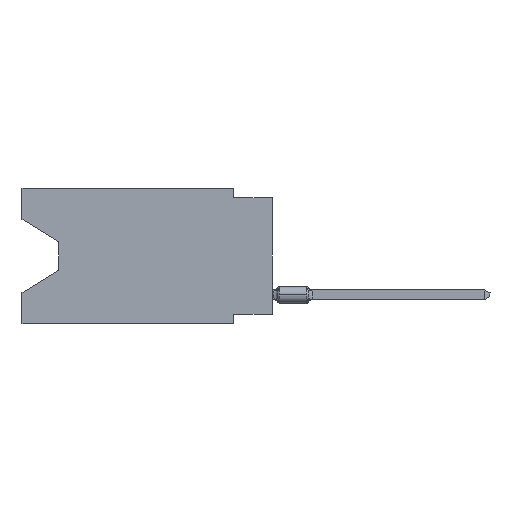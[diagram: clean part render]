
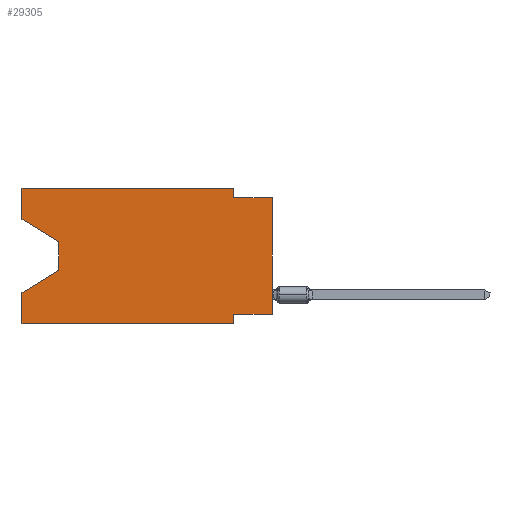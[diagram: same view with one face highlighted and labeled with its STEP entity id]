
A CAD part, left-side view. The second image highlights one B-rep face of the part: STEP entity #29305.
In plain terms, the highlighted planar face has unit normal (-1, 0, 0).
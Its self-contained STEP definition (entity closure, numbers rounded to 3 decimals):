
#318 = DIRECTION ( 'NONE',  ( 0., 0., -1. ) ) ;
#501 = VERTEX_POINT ( 'NONE', #9343 ) ;
#638 = CARTESIAN_POINT ( 'NONE',  ( 0., 0., -8.255 ) ) ;
#1353 = LINE ( 'NONE', #30160, #41318 ) ;
#1791 = VERTEX_POINT ( 'NONE', #24906 ) ;
#1804 = VERTEX_POINT ( 'NONE', #42028 ) ;
#1901 = VECTOR ( 'NONE', #5568, 1000. ) ;
#2150 = ORIENTED_EDGE ( 'NONE', *, *, #16579, .F. ) ;
#2250 = EDGE_CURVE ( 'NONE', #501, #45289, #46612, .T. ) ;
#2260 = CARTESIAN_POINT ( 'NONE',  ( 0., 0., 0. ) ) ;
#2474 = LINE ( 'NONE', #16874, #13094 ) ;
#3110 = DIRECTION ( 'NONE',  ( 1., 0., 0. ) ) ;
#3567 = LINE ( 'NONE', #17994, #26788 ) ;
#4320 = EDGE_CURVE ( 'NONE', #13395, #40575, #29215, .T. ) ;
#4702 = VECTOR ( 'NONE', #33225, 1000. ) ;
#4953 = CARTESIAN_POINT ( 'NONE',  ( 0., 2.54, -8.89 ) ) ;
#5279 = ORIENTED_EDGE ( 'NONE', *, *, #11830, .F. ) ;
#5568 = DIRECTION ( 'NONE',  ( 0., 0., 1. ) ) ;
#6064 = CARTESIAN_POINT ( 'NONE',  ( 0., 0., -8.255 ) ) ;
#6344 = CARTESIAN_POINT ( 'NONE',  ( 0., 16.383, -8.89 ) ) ;
#7563 = VECTOR ( 'NONE', #28225, 1000. ) ;
#7940 = DIRECTION ( 'NONE',  ( 0., 1., 0. ) ) ;
#8797 = VECTOR ( 'NONE', #27141, 1000. ) ;
#9343 = CARTESIAN_POINT ( 'NONE',  ( 0., 16.383, -2.038 ) ) ;
#9358 = DIRECTION ( 'NONE',  ( 0., 0.855, -0.519 ) ) ;
#10024 = LINE ( 'NONE', #21334, #24580 ) ;
#10184 = VECTOR ( 'NONE', #20744, 1000. ) ;
#10785 = DIRECTION ( 'NONE',  ( 0., 0., -1. ) ) ;
#11239 = ORIENTED_EDGE ( 'NONE', *, *, #15817, .F. ) ;
#11830 = EDGE_CURVE ( 'NONE', #44606, #1804, #18575, .T. ) ;
#12514 = CARTESIAN_POINT ( 'NONE',  ( 0., 16.383, 0. ) ) ;
#13094 = VECTOR ( 'NONE', #14985, 1000. ) ;
#13395 = VERTEX_POINT ( 'NONE', #42194 ) ;
#13863 = CARTESIAN_POINT ( 'NONE',  ( 0., 2.54, -8.89 ) ) ;
#13986 = FACE_OUTER_BOUND ( 'NONE', #30178, .T. ) ;
#14334 = AXIS2_PLACEMENT_3D ( 'NONE', #35450, #3110, #39457 ) ;
#14600 = EDGE_CURVE ( 'NONE', #44606, #38113, #16658, .T. ) ;
#14623 = EDGE_CURVE ( 'NONE', #40575, #28723, #3567, .T. ) ;
#14646 = ORIENTED_EDGE ( 'NONE', *, *, #37536, .F. ) ;
#14985 = DIRECTION ( 'NONE',  ( 0., -1., 0. ) ) ;
#15817 = EDGE_CURVE ( 'NONE', #28723, #38113, #2474, .T. ) ;
#16579 = EDGE_CURVE ( 'NONE', #1804, #25787, #42405, .T. ) ;
#16658 = LINE ( 'NONE', #2260, #1901 ) ;
#16874 = CARTESIAN_POINT ( 'NONE',  ( 0., 0., -0.635 ) ) ;
#17994 = CARTESIAN_POINT ( 'NONE',  ( 0., 2.54, 0. ) ) ;
#18475 = ORIENTED_EDGE ( 'NONE', *, *, #20558, .T. ) ;
#18575 = LINE ( 'NONE', #638, #31846 ) ;
#19889 = LINE ( 'NONE', #44659, #41288 ) ;
#20558 = EDGE_CURVE ( 'NONE', #45289, #23572, #10024, .T. ) ;
#20721 = ORIENTED_EDGE ( 'NONE', *, *, #4320, .F. ) ;
#20744 = DIRECTION ( 'NONE',  ( 0., -1., 0. ) ) ;
#21334 = CARTESIAN_POINT ( 'NONE',  ( 0., 13.97, -3.505 ) ) ;
#21909 = CARTESIAN_POINT ( 'NONE',  ( 0., 16.383, 0. ) ) ;
#23572 = VERTEX_POINT ( 'NONE', #41243 ) ;
#24580 = VECTOR ( 'NONE', #318, 1000. ) ;
#24906 = CARTESIAN_POINT ( 'NONE',  ( 0., 16.383, -8.89 ) ) ;
#24958 = EDGE_CURVE ( 'NONE', #501, #13395, #26904, .T. ) ;
#25787 = VERTEX_POINT ( 'NONE', #4953 ) ;
#25959 = VECTOR ( 'NONE', #10785, 1000. ) ;
#26788 = VECTOR ( 'NONE', #32383, 1000. ) ;
#26904 = LINE ( 'NONE', #12514, #8797 ) ;
#27141 = DIRECTION ( 'NONE',  ( 0., 0., 1. ) ) ;
#27263 = EDGE_CURVE ( 'NONE', #23572, #31682, #1353, .T. ) ;
#27689 = PLANE ( 'NONE',  #14334 ) ;
#27996 = ORIENTED_EDGE ( 'NONE', *, *, #2250, .T. ) ;
#28225 = DIRECTION ( 'NONE',  ( 0., -0.855, -0.519 ) ) ;
#28232 = CARTESIAN_POINT ( 'NONE',  ( 0., 0., -0.635 ) ) ;
#28723 = VERTEX_POINT ( 'NONE', #41277 ) ;
#29215 = LINE ( 'NONE', #21909, #4702 ) ;
#29305 = ADVANCED_FACE ( 'NONE', ( #13986 ), #27689, .F. ) ;
#30160 = CARTESIAN_POINT ( 'NONE',  ( 0., 13.97, -5.385 ) ) ;
#30178 = EDGE_LOOP ( 'NONE', ( #27996, #18475, #34862, #14646, #35915, #2150, #5279, #32126, #11239, #42707, #20721, #45564 ) ) ;
#31483 = CARTESIAN_POINT ( 'NONE',  ( 0., 16.383, -6.852 ) ) ;
#31682 = VERTEX_POINT ( 'NONE', #31483 ) ;
#31846 = VECTOR ( 'NONE', #7940, 1000. ) ;
#32126 = ORIENTED_EDGE ( 'NONE', *, *, #14600, .T. ) ;
#32360 = CARTESIAN_POINT ( 'NONE',  ( 0., 2.54, 0. ) ) ;
#32383 = DIRECTION ( 'NONE',  ( 0., 0., -1. ) ) ;
#33225 = DIRECTION ( 'NONE',  ( 0., -1., 0. ) ) ;
#34862 = ORIENTED_EDGE ( 'NONE', *, *, #27263, .T. ) ;
#35450 = CARTESIAN_POINT ( 'NONE',  ( 0., 16.383, 0. ) ) ;
#35915 = ORIENTED_EDGE ( 'NONE', *, *, #40968, .T. ) ;
#36413 = CARTESIAN_POINT ( 'NONE',  ( 0., 13.97, -3.505 ) ) ;
#37536 = EDGE_CURVE ( 'NONE', #1791, #31682, #19889, .T. ) ;
#38113 = VERTEX_POINT ( 'NONE', #28232 ) ;
#39457 = DIRECTION ( 'NONE',  ( 0., 0., -1. ) ) ;
#40575 = VERTEX_POINT ( 'NONE', #32360 ) ;
#40968 = EDGE_CURVE ( 'NONE', #1791, #25787, #46205, .T. ) ;
#41243 = CARTESIAN_POINT ( 'NONE',  ( 0., 13.97, -5.385 ) ) ;
#41277 = CARTESIAN_POINT ( 'NONE',  ( 0., 2.54, -0.635 ) ) ;
#41288 = VECTOR ( 'NONE', #43969, 1000. ) ;
#41318 = VECTOR ( 'NONE', #9358, 1000. ) ;
#42028 = CARTESIAN_POINT ( 'NONE',  ( 0., 2.54, -8.255 ) ) ;
#42194 = CARTESIAN_POINT ( 'NONE',  ( 0., 16.383, 0. ) ) ;
#42405 = LINE ( 'NONE', #13863, #25959 ) ;
#42707 = ORIENTED_EDGE ( 'NONE', *, *, #14623, .F. ) ;
#43068 = CARTESIAN_POINT ( 'NONE',  ( 0., 16.383, -2.038 ) ) ;
#43969 = DIRECTION ( 'NONE',  ( 0., 0., 1. ) ) ;
#44606 = VERTEX_POINT ( 'NONE', #6064 ) ;
#44659 = CARTESIAN_POINT ( 'NONE',  ( 0., 16.383, 0. ) ) ;
#45289 = VERTEX_POINT ( 'NONE', #36413 ) ;
#45564 = ORIENTED_EDGE ( 'NONE', *, *, #24958, .F. ) ;
#46205 = LINE ( 'NONE', #6344, #10184 ) ;
#46612 = LINE ( 'NONE', #43068, #7563 ) ;
